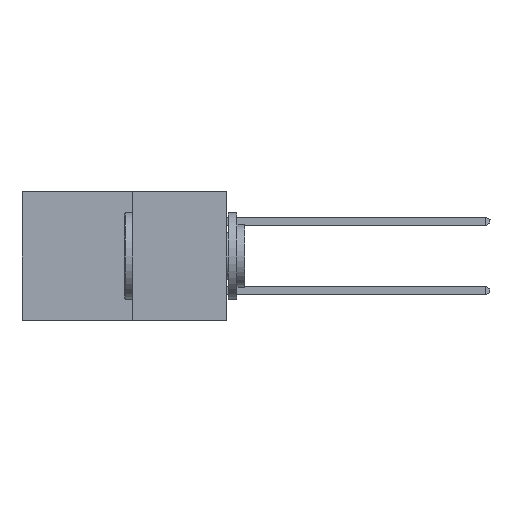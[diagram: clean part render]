
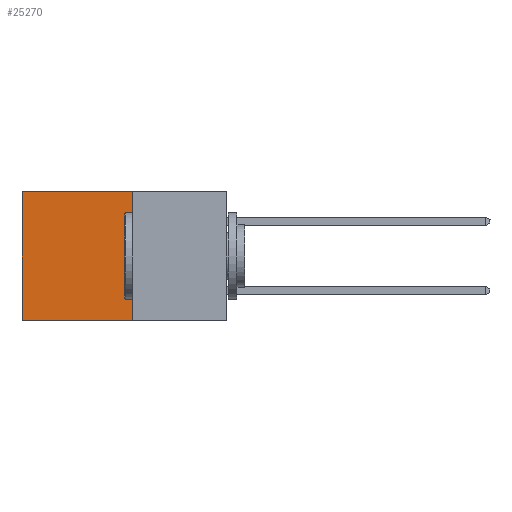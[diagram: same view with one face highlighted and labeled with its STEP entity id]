
A CAD part, left-side view. The second image highlights one B-rep face of the part: STEP entity #25270.
In plain terms, the highlighted planar face has unit normal (-1, 0, 0).
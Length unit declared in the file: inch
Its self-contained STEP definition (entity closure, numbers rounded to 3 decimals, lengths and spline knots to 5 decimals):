
#32 = ORIENTED_EDGE ( 'NONE', *, *, #5137, .T. ) ;
#370 = EDGE_CURVE ( 'NONE', #1522, #3183, #3970, .T. ) ;
#778 = LINE ( 'NONE', #19168, #6887 ) ;
#1522 = VERTEX_POINT ( 'NONE', #28525 ) ;
#3183 = VERTEX_POINT ( 'NONE', #29763 ) ;
#3674 = DIRECTION ( 'NONE',  ( 0., 0., -1. ) ) ;
#3970 = LINE ( 'NONE', #18723, #22986 ) ;
#5137 = EDGE_CURVE ( 'NONE', #20457, #33183, #22553, .T. ) ;
#6887 = VECTOR ( 'NONE', #3674, 39.37008 ) ;
#7419 = ORIENTED_EDGE ( 'NONE', *, *, #28393, .F. ) ;
#11417 = CARTESIAN_POINT ( 'NONE',  ( 0.277, 0.59, 0. ) ) ;
#14846 = VECTOR ( 'NONE', #26115, 39.37008 ) ;
#15235 = DIRECTION ( 'NONE',  ( 1., 0., 0. ) ) ;
#15439 = ORIENTED_EDGE ( 'NONE', *, *, #30761, .T. ) ;
#15552 = ORIENTED_EDGE ( 'NONE', *, *, #370, .F. ) ;
#16840 = LINE ( 'NONE', #30276, #23714 ) ;
#18723 = CARTESIAN_POINT ( 'NONE',  ( 0.277, 0.27, -0.37 ) ) ;
#19168 = CARTESIAN_POINT ( 'NONE',  ( 0.277, 0.27, -0.37 ) ) ;
#20457 = VERTEX_POINT ( 'NONE', #30647 ) ;
#21507 = EDGE_LOOP ( 'NONE', ( #15439, #15552, #7419, #32 ) ) ;
#22553 = LINE ( 'NONE', #24722, #14846 ) ;
#22942 = PLANE ( 'NONE',  #23000 ) ;
#22986 = VECTOR ( 'NONE', #29414, 39.37008 ) ;
#23000 = AXIS2_PLACEMENT_3D ( 'NONE', #30577, #15235, #33091 ) ;
#23714 = VECTOR ( 'NONE', #25296, 39.37008 ) ;
#23806 = FACE_OUTER_BOUND ( 'NONE', #21507, .T. ) ;
#24722 = CARTESIAN_POINT ( 'NONE',  ( 0.277, 0.27, 0. ) ) ;
#25270 = ADVANCED_FACE ( 'NONE', ( #23806 ), #22942, .F. ) ;
#25296 = DIRECTION ( 'NONE',  ( 0., 0., -1. ) ) ;
#26115 = DIRECTION ( 'NONE',  ( 0., 1., 0. ) ) ;
#28393 = EDGE_CURVE ( 'NONE', #20457, #1522, #778, .T. ) ;
#28525 = CARTESIAN_POINT ( 'NONE',  ( 0.277, 0.27, -0.37 ) ) ;
#29414 = DIRECTION ( 'NONE',  ( 0., 1., 0. ) ) ;
#29763 = CARTESIAN_POINT ( 'NONE',  ( 0.277, 0.59, -0.37 ) ) ;
#30276 = CARTESIAN_POINT ( 'NONE',  ( 0.277, 0.59, -0.37 ) ) ;
#30577 = CARTESIAN_POINT ( 'NONE',  ( 0.277, 0.27, -0.37 ) ) ;
#30647 = CARTESIAN_POINT ( 'NONE',  ( 0.277, 0.27, 0. ) ) ;
#30761 = EDGE_CURVE ( 'NONE', #33183, #3183, #16840, .T. ) ;
#33091 = DIRECTION ( 'NONE',  ( 0., 0., -1. ) ) ;
#33183 = VERTEX_POINT ( 'NONE', #11417 ) ;
